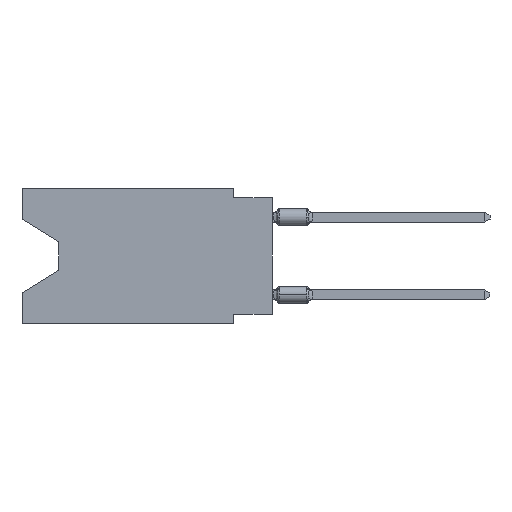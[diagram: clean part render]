
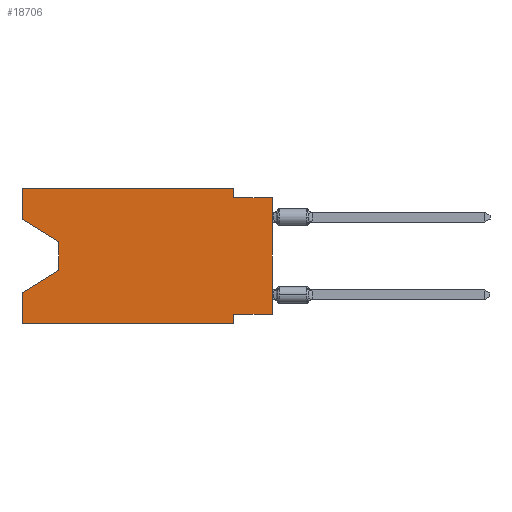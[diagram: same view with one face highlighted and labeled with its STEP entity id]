
A CAD part, left-side view. The second image highlights one B-rep face of the part: STEP entity #18706.
In plain terms, the highlighted planar face has unit normal (-1, 0, 0).
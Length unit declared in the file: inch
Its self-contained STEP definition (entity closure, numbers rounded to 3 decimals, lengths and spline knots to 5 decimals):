
#720 = CARTESIAN_POINT ( 'NONE',  ( 0., 0.645, 0. ) ) ;
#1357 = VECTOR ( 'NONE', #25586, 39.37008 ) ;
#1363 = ORIENTED_EDGE ( 'NONE', *, *, #21067, .F. ) ;
#1649 = CARTESIAN_POINT ( 'NONE',  ( 0., 0.55, -0.138 ) ) ;
#1729 = DIRECTION ( 'NONE',  ( 0., 0., 1. ) ) ;
#2161 = EDGE_CURVE ( 'NONE', #19979, #25843, #3190, .T. ) ;
#2972 = CARTESIAN_POINT ( 'NONE',  ( 0., 0.55, -0.138 ) ) ;
#3190 = LINE ( 'NONE', #14331, #40508 ) ;
#3827 = DIRECTION ( 'NONE',  ( 0., -1., 0. ) ) ;
#4235 = VERTEX_POINT ( 'NONE', #41013 ) ;
#4384 = EDGE_CURVE ( 'NONE', #4235, #41808, #9781, .T. ) ;
#4911 = ORIENTED_EDGE ( 'NONE', *, *, #21931, .T. ) ;
#5130 = VERTEX_POINT ( 'NONE', #27337 ) ;
#5654 = VERTEX_POINT ( 'NONE', #8624 ) ;
#5987 = ORIENTED_EDGE ( 'NONE', *, *, #34316, .F. ) ;
#6010 = ORIENTED_EDGE ( 'NONE', *, *, #2161, .F. ) ;
#6034 = DIRECTION ( 'NONE',  ( 0., 0., -1. ) ) ;
#6437 = LINE ( 'NONE', #20894, #13215 ) ;
#6484 = CARTESIAN_POINT ( 'NONE',  ( 0., 0., -0.025 ) ) ;
#6641 = DIRECTION ( 'NONE',  ( 0., -0.855, -0.519 ) ) ;
#6818 = CARTESIAN_POINT ( 'NONE',  ( 0., 0.645, -0.35 ) ) ;
#7382 = CARTESIAN_POINT ( 'NONE',  ( 0., 0.645, 0. ) ) ;
#7480 = EDGE_CURVE ( 'NONE', #4235, #19979, #26953, .T. ) ;
#7625 = DIRECTION ( 'NONE',  ( 1., 0., 0. ) ) ;
#8624 = CARTESIAN_POINT ( 'NONE',  ( 0., 0.645, -0.08025 ) ) ;
#9275 = VECTOR ( 'NONE', #24839, 39.37008 ) ;
#9676 = VECTOR ( 'NONE', #6641, 39.37008 ) ;
#9781 = LINE ( 'NONE', #20650, #19390 ) ;
#9784 = VECTOR ( 'NONE', #41374, 39.37008 ) ;
#9987 = CARTESIAN_POINT ( 'NONE',  ( 0., 0., -0.025 ) ) ;
#10970 = ORIENTED_EDGE ( 'NONE', *, *, #33779, .F. ) ;
#11617 = VERTEX_POINT ( 'NONE', #2972 ) ;
#12427 = ORIENTED_EDGE ( 'NONE', *, *, #23526, .F. ) ;
#12877 = EDGE_CURVE ( 'NONE', #5130, #25843, #21726, .T. ) ;
#13215 = VECTOR ( 'NONE', #1729, 39.37008 ) ;
#14331 = CARTESIAN_POINT ( 'NONE',  ( 0., 0.1, -0.35 ) ) ;
#14942 = VECTOR ( 'NONE', #32818, 39.37008 ) ;
#15255 = CARTESIAN_POINT ( 'NONE',  ( 0., 0.645, -0.26975 ) ) ;
#17552 = LINE ( 'NONE', #9987, #26061 ) ;
#17912 = VERTEX_POINT ( 'NONE', #23159 ) ;
#18706 = ADVANCED_FACE ( 'NONE', ( #44069 ), #18986, .F. ) ;
#18986 = PLANE ( 'NONE',  #28135 ) ;
#19390 = VECTOR ( 'NONE', #45993, 39.37008 ) ;
#19909 = ORIENTED_EDGE ( 'NONE', *, *, #30078, .T. ) ;
#19979 = VERTEX_POINT ( 'NONE', #39277 ) ;
#20047 = CARTESIAN_POINT ( 'NONE',  ( 0., 0.1, 0. ) ) ;
#20650 = CARTESIAN_POINT ( 'NONE',  ( 0., 0., 0. ) ) ;
#20894 = CARTESIAN_POINT ( 'NONE',  ( 0., 0.645, 0. ) ) ;
#21067 = EDGE_CURVE ( 'NONE', #43660, #24575, #22987, .T. ) ;
#21726 = LINE ( 'NONE', #6818, #14942 ) ;
#21825 = LINE ( 'NONE', #28899, #32119 ) ;
#21931 = EDGE_CURVE ( 'NONE', #17912, #26404, #21825, .T. ) ;
#22987 = LINE ( 'NONE', #36937, #40397 ) ;
#23159 = CARTESIAN_POINT ( 'NONE',  ( 0., 0.55, -0.212 ) ) ;
#23417 = CARTESIAN_POINT ( 'NONE',  ( 0., 0., -0.325 ) ) ;
#23526 = EDGE_CURVE ( 'NONE', #5130, #26404, #6437, .T. ) ;
#24027 = ORIENTED_EDGE ( 'NONE', *, *, #4384, .T. ) ;
#24385 = VERTEX_POINT ( 'NONE', #30635 ) ;
#24575 = VERTEX_POINT ( 'NONE', #25421 ) ;
#24645 = LINE ( 'NONE', #39060, #9676 ) ;
#24839 = DIRECTION ( 'NONE',  ( 0., 0., -1. ) ) ;
#25421 = CARTESIAN_POINT ( 'NONE',  ( 0., 0.1, 0. ) ) ;
#25586 = DIRECTION ( 'NONE',  ( 0., 0., 1. ) ) ;
#25843 = VERTEX_POINT ( 'NONE', #43715 ) ;
#26061 = VECTOR ( 'NONE', #28878, 39.37008 ) ;
#26404 = VERTEX_POINT ( 'NONE', #15255 ) ;
#26953 = LINE ( 'NONE', #23417, #9784 ) ;
#27337 = CARTESIAN_POINT ( 'NONE',  ( 0., 0.645, -0.35 ) ) ;
#27422 = ORIENTED_EDGE ( 'NONE', *, *, #12877, .T. ) ;
#28135 = AXIS2_PLACEMENT_3D ( 'NONE', #7382, #7625, #29613 ) ;
#28293 = ORIENTED_EDGE ( 'NONE', *, *, #43735, .F. ) ;
#28878 = DIRECTION ( 'NONE',  ( 0., -1., 0. ) ) ;
#28899 = CARTESIAN_POINT ( 'NONE',  ( 0., 0.55, -0.212 ) ) ;
#29613 = DIRECTION ( 'NONE',  ( 0., 0., -1. ) ) ;
#30078 = EDGE_CURVE ( 'NONE', #11617, #17912, #41165, .T. ) ;
#30635 = CARTESIAN_POINT ( 'NONE',  ( 0., 0.1, -0.025 ) ) ;
#32119 = VECTOR ( 'NONE', #36470, 39.37008 ) ;
#32818 = DIRECTION ( 'NONE',  ( 0., -1., 0. ) ) ;
#33068 = VECTOR ( 'NONE', #38012, 39.37008 ) ;
#33726 = ORIENTED_EDGE ( 'NONE', *, *, #34266, .T. ) ;
#33779 = EDGE_CURVE ( 'NONE', #24575, #24385, #34925, .T. ) ;
#34266 = EDGE_CURVE ( 'NONE', #5654, #11617, #24645, .T. ) ;
#34316 = EDGE_CURVE ( 'NONE', #5654, #43660, #36451, .T. ) ;
#34925 = LINE ( 'NONE', #20047, #33068 ) ;
#35621 = EDGE_LOOP ( 'NONE', ( #33726, #19909, #4911, #12427, #27422, #6010, #37171, #24027, #28293, #10970, #1363, #5987 ) ) ;
#36451 = LINE ( 'NONE', #720, #1357 ) ;
#36470 = DIRECTION ( 'NONE',  ( 0., 0.855, -0.519 ) ) ;
#36937 = CARTESIAN_POINT ( 'NONE',  ( 0., 0.645, 0. ) ) ;
#37171 = ORIENTED_EDGE ( 'NONE', *, *, #7480, .F. ) ;
#38012 = DIRECTION ( 'NONE',  ( 0., 0., -1. ) ) ;
#39060 = CARTESIAN_POINT ( 'NONE',  ( 0., 0.645, -0.08025 ) ) ;
#39277 = CARTESIAN_POINT ( 'NONE',  ( 0., 0.1, -0.325 ) ) ;
#40397 = VECTOR ( 'NONE', #3827, 39.37008 ) ;
#40508 = VECTOR ( 'NONE', #6034, 39.37008 ) ;
#41013 = CARTESIAN_POINT ( 'NONE',  ( 0., 0., -0.325 ) ) ;
#41165 = LINE ( 'NONE', #1649, #9275 ) ;
#41374 = DIRECTION ( 'NONE',  ( 0., 1., 0. ) ) ;
#41670 = CARTESIAN_POINT ( 'NONE',  ( 0., 0.645, 0. ) ) ;
#41808 = VERTEX_POINT ( 'NONE', #6484 ) ;
#43660 = VERTEX_POINT ( 'NONE', #41670 ) ;
#43715 = CARTESIAN_POINT ( 'NONE',  ( 0., 0.1, -0.35 ) ) ;
#43735 = EDGE_CURVE ( 'NONE', #24385, #41808, #17552, .T. ) ;
#44069 = FACE_OUTER_BOUND ( 'NONE', #35621, .T. ) ;
#45993 = DIRECTION ( 'NONE',  ( 0., 0., 1. ) ) ;
